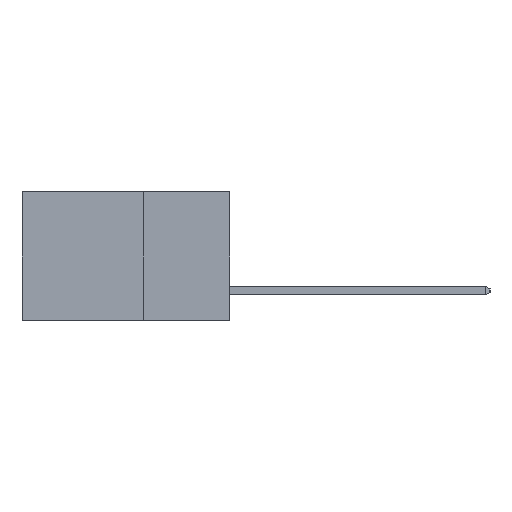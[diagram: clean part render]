
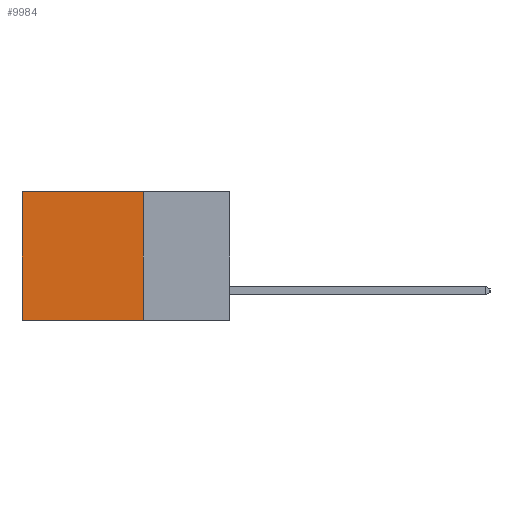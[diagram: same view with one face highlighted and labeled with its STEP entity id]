
A CAD part, left-side view. The second image highlights one B-rep face of the part: STEP entity #9984.
In plain terms, the highlighted planar face has unit normal (-1, 0, 0).
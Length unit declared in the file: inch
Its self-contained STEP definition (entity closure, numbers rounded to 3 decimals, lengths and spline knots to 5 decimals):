
#592 = VECTOR ( 'NONE', #4973, 39.37008 ) ;
#965 = VECTOR ( 'NONE', #7984, 39.37008 ) ;
#1097 = CARTESIAN_POINT ( 'NONE',  ( 0.2615, 0.25, -0.37 ) ) ;
#1726 = VECTOR ( 'NONE', #2851, 39.37008 ) ;
#1751 = DIRECTION ( 'NONE',  ( 0., 0., -1. ) ) ;
#1787 = DIRECTION ( 'NONE',  ( 1., 0., 0. ) ) ;
#1796 = ORIENTED_EDGE ( 'NONE', *, *, #2295, .T. ) ;
#1800 = PLANE ( 'NONE',  #5611 ) ;
#2158 = CARTESIAN_POINT ( 'NONE',  ( 0.2615, 0.25, -0.37 ) ) ;
#2295 = EDGE_CURVE ( 'NONE', #5489, #7124, #3547, .T. ) ;
#2414 = LINE ( 'NONE', #4871, #592 ) ;
#2756 = EDGE_LOOP ( 'NONE', ( #1796, #5303, #3236, #8356 ) ) ;
#2851 = DIRECTION ( 'NONE',  ( 0., 1., 0. ) ) ;
#3121 = VERTEX_POINT ( 'NONE', #3719 ) ;
#3155 = EDGE_CURVE ( 'NONE', #3121, #5489, #3527, .T. ) ;
#3236 = ORIENTED_EDGE ( 'NONE', *, *, #9834, .F. ) ;
#3527 = LINE ( 'NONE', #5901, #8173 ) ;
#3547 = LINE ( 'NONE', #8109, #965 ) ;
#3719 = CARTESIAN_POINT ( 'NONE',  ( 0.2615, 0.25, 0. ) ) ;
#4031 = CARTESIAN_POINT ( 'NONE',  ( 0.2615, 0.6, -0.37 ) ) ;
#4871 = CARTESIAN_POINT ( 'NONE',  ( 0.2615, 0.25, -0.37 ) ) ;
#4943 = VERTEX_POINT ( 'NONE', #7011 ) ;
#4973 = DIRECTION ( 'NONE',  ( 0., 0., -1. ) ) ;
#5303 = ORIENTED_EDGE ( 'NONE', *, *, #10091, .F. ) ;
#5489 = VERTEX_POINT ( 'NONE', #7814 ) ;
#5611 = AXIS2_PLACEMENT_3D ( 'NONE', #2158, #1787, #1751 ) ;
#5901 = CARTESIAN_POINT ( 'NONE',  ( 0.2615, 0.25, 0. ) ) ;
#6725 = DIRECTION ( 'NONE',  ( 0., 1., 0. ) ) ;
#7011 = CARTESIAN_POINT ( 'NONE',  ( 0.2615, 0.25, -0.37 ) ) ;
#7124 = VERTEX_POINT ( 'NONE', #4031 ) ;
#7814 = CARTESIAN_POINT ( 'NONE',  ( 0.2615, 0.6, 0. ) ) ;
#7984 = DIRECTION ( 'NONE',  ( 0., 0., -1. ) ) ;
#8109 = CARTESIAN_POINT ( 'NONE',  ( 0.2615, 0.6, -0.37 ) ) ;
#8173 = VECTOR ( 'NONE', #6725, 39.37008 ) ;
#8356 = ORIENTED_EDGE ( 'NONE', *, *, #3155, .T. ) ;
#9349 = FACE_OUTER_BOUND ( 'NONE', #2756, .T. ) ;
#9834 = EDGE_CURVE ( 'NONE', #3121, #4943, #2414, .T. ) ;
#9984 = ADVANCED_FACE ( 'NONE', ( #9349 ), #1800, .F. ) ;
#10091 = EDGE_CURVE ( 'NONE', #4943, #7124, #10191, .T. ) ;
#10191 = LINE ( 'NONE', #1097, #1726 ) ;
